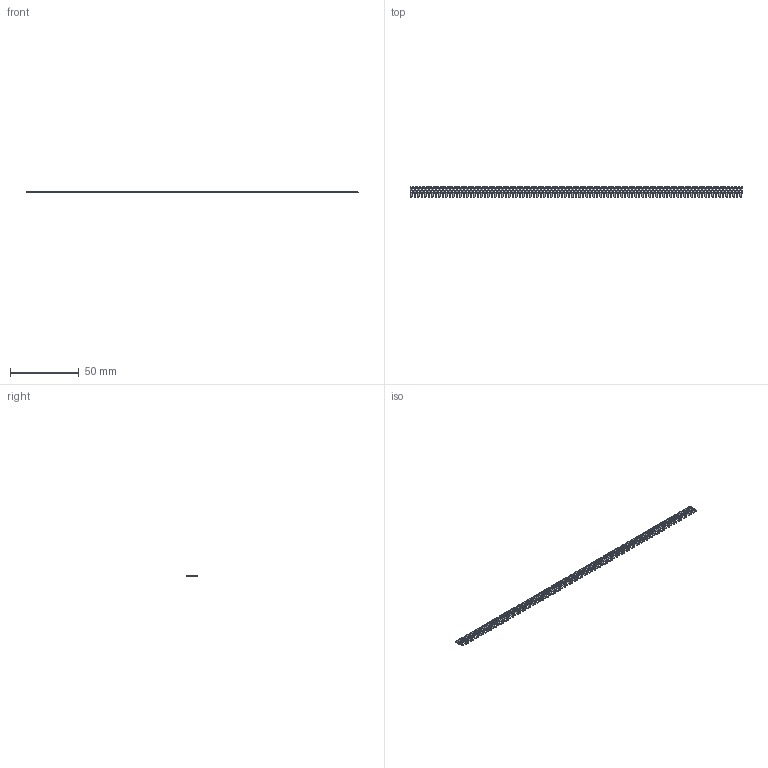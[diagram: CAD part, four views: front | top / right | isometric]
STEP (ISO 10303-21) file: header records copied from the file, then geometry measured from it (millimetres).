
FILE_DESCRIPTION (( 'STEP AP203' ), '1' );
FILE_NAME ('103-095-253-100.STEP', '2020-04-16T17:15:57', ( '' ), ( '' ), 'SwSTEP 2.0', 'SolidWorks 2016', '' );
FILE_SCHEMA (( 'CONFIG_CONTROL_DESIGN' ));
Length unit declared in the file: inch
Products named in the file (2): 103-095-253-100; 100-290-001_100-290-253
Assembly tree (95 placements, depth 2):
  103-095-253-100
    100-290-001_100-290-253  x95
Bounding box: 240.79 x 7.62 x 0.51 mm (x, y, z)
Volume: 524.2 mm3; surface area: 3268.7 mm2
Topology: 95 solids, 95 shells, 1900 faces, 5130 edges, 3420 vertices
Faces by surface type: plane 1805, cylinder 95
Entity records: 3828 total; most frequent: DIRECTION 292, CARTESIAN_POINT 208, COORDINATED_UNIVERSAL_TIME_OFFSET 200, LOCAL_TIME 200, DATE_AND_TIME 200, CALENDAR_DATE 200, AXIS2_PLACEMENT_3D 120, PERSON_AND_ORGANIZATION 111
